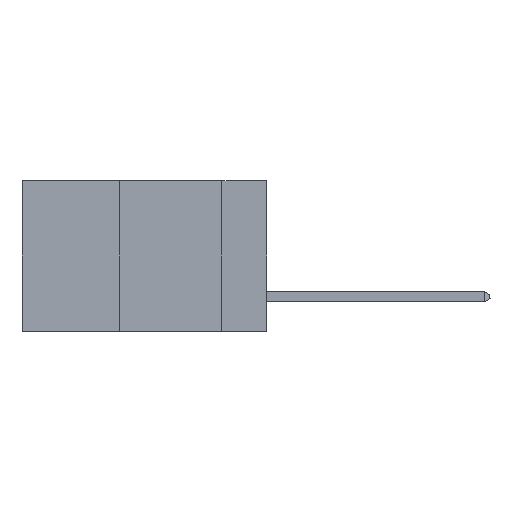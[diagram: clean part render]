
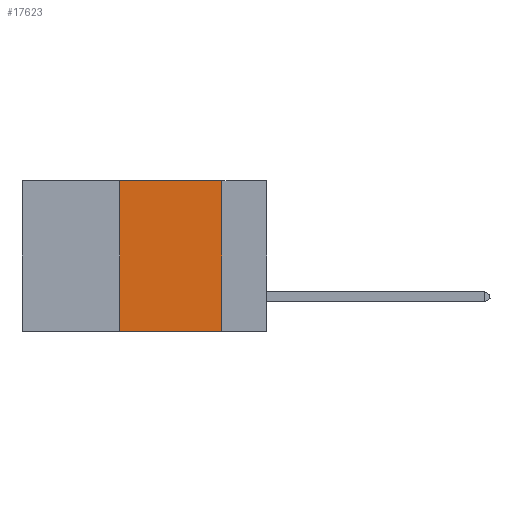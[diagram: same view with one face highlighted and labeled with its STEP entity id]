
A CAD part, left-side view. The second image highlights one B-rep face of the part: STEP entity #17623.
In plain terms, the highlighted planar face has unit normal (-1, 0, 0).
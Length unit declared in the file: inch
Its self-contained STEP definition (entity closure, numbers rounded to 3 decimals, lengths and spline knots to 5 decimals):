
#494 = DIRECTION ( 'NONE',  ( 1., 0., 0. ) ) ;
#1000 = VECTOR ( 'NONE', #1350, 39.37008 ) ;
#1350 = DIRECTION ( 'NONE',  ( 0., 0., 1. ) ) ;
#1669 = EDGE_CURVE ( 'NONE', #19197, #15132, #15362, .T. ) ;
#3122 = VECTOR ( 'NONE', #3531, 39.37008 ) ;
#3531 = DIRECTION ( 'NONE',  ( 0., 0., -1. ) ) ;
#4111 = EDGE_CURVE ( 'NONE', #20704, #12843, #17386, .T. ) ;
#4205 = EDGE_CURVE ( 'NONE', #19197, #20704, #12397, .T. ) ;
#4792 = VECTOR ( 'NONE', #15921, 39.37008 ) ;
#5367 = DIRECTION ( 'NONE',  ( 0., -1., 0. ) ) ;
#5482 = CARTESIAN_POINT ( 'NONE',  ( 0., 0.11, 0. ) ) ;
#5513 = VECTOR ( 'NONE', #5367, 39.37008 ) ;
#5544 = CARTESIAN_POINT ( 'NONE',  ( 0., 0.6, 0. ) ) ;
#5602 = FACE_OUTER_BOUND ( 'NONE', #8803, .T. ) ;
#5787 = LINE ( 'NONE', #8699, #3122 ) ;
#7943 = ORIENTED_EDGE ( 'NONE', *, *, #4205, .F. ) ;
#8699 = CARTESIAN_POINT ( 'NONE',  ( 0., 0.11, 0. ) ) ;
#8803 = EDGE_LOOP ( 'NONE', ( #21401, #16088, #7943, #16143 ) ) ;
#11521 = CARTESIAN_POINT ( 'NONE',  ( 0., 0.6, 0. ) ) ;
#11619 = CARTESIAN_POINT ( 'NONE',  ( 0., 0.36, -0.37 ) ) ;
#12397 = LINE ( 'NONE', #15983, #1000 ) ;
#12843 = VERTEX_POINT ( 'NONE', #5482 ) ;
#14378 = CARTESIAN_POINT ( 'NONE',  ( 0., 0.11, -0.37 ) ) ;
#15132 = VERTEX_POINT ( 'NONE', #14378 ) ;
#15362 = LINE ( 'NONE', #17482, #4792 ) ;
#15921 = DIRECTION ( 'NONE',  ( 0., -1., 0. ) ) ;
#15983 = CARTESIAN_POINT ( 'NONE',  ( 0., 0.36, 0. ) ) ;
#16088 = ORIENTED_EDGE ( 'NONE', *, *, #4111, .F. ) ;
#16143 = ORIENTED_EDGE ( 'NONE', *, *, #1669, .T. ) ;
#17345 = DIRECTION ( 'NONE',  ( 0., 0., -1. ) ) ;
#17386 = LINE ( 'NONE', #11521, #5513 ) ;
#17482 = CARTESIAN_POINT ( 'NONE',  ( 0., 0.6, -0.37 ) ) ;
#17497 = PLANE ( 'NONE',  #21874 ) ;
#17623 = ADVANCED_FACE ( 'NONE', ( #5602 ), #17497, .F. ) ;
#18098 = CARTESIAN_POINT ( 'NONE',  ( 0., 0.36, 0. ) ) ;
#19197 = VERTEX_POINT ( 'NONE', #11619 ) ;
#20704 = VERTEX_POINT ( 'NONE', #18098 ) ;
#20959 = EDGE_CURVE ( 'NONE', #12843, #15132, #5787, .T. ) ;
#21401 = ORIENTED_EDGE ( 'NONE', *, *, #20959, .F. ) ;
#21874 = AXIS2_PLACEMENT_3D ( 'NONE', #5544, #494, #17345 ) ;
